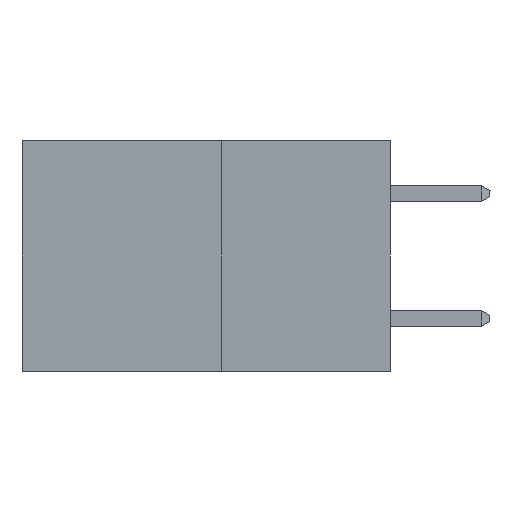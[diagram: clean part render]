
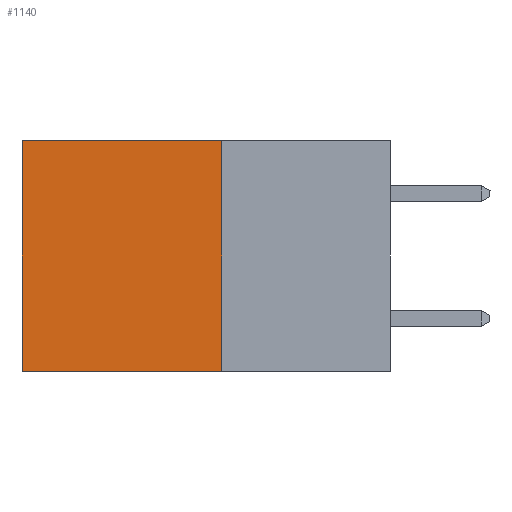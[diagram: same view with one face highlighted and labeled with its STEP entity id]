
A CAD part, left-side view. The second image highlights one B-rep face of the part: STEP entity #1140.
In plain terms, the highlighted planar face has unit normal (-1, 0, 0).
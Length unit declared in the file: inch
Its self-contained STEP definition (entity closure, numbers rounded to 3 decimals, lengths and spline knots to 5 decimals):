
#86 = CARTESIAN_POINT ( 'NONE',  ( 0.277, 0.59, -0.37 ) ) ;
#285 = CARTESIAN_POINT ( 'NONE',  ( 0.277, 0.27, 0. ) ) ;
#1140 = ADVANCED_FACE ( 'NONE', ( #10723 ), #2775, .F. ) ;
#1221 = VECTOR ( 'NONE', #5874, 39.37008 ) ;
#1782 = EDGE_CURVE ( 'NONE', #11615, #2696, #5138, .T. ) ;
#1814 = CARTESIAN_POINT ( 'NONE',  ( 0.277, 0.59, 0. ) ) ;
#1834 = ORIENTED_EDGE ( 'NONE', *, *, #4862, .T. ) ;
#2696 = VERTEX_POINT ( 'NONE', #1814 ) ;
#2775 = PLANE ( 'NONE',  #9200 ) ;
#2791 = EDGE_CURVE ( 'NONE', #6132, #6072, #4108, .T. ) ;
#2902 = CARTESIAN_POINT ( 'NONE',  ( 0.277, 0.27, -0.37 ) ) ;
#4064 = ORIENTED_EDGE ( 'NONE', *, *, #2791, .F. ) ;
#4078 = ORIENTED_EDGE ( 'NONE', *, *, #4634, .F. ) ;
#4108 = LINE ( 'NONE', #11691, #8638 ) ;
#4379 = VECTOR ( 'NONE', #5209, 39.37008 ) ;
#4634 = EDGE_CURVE ( 'NONE', #11615, #6132, #10956, .T. ) ;
#4862 = EDGE_CURVE ( 'NONE', #2696, #6072, #6765, .T. ) ;
#5138 = LINE ( 'NONE', #11269, #7789 ) ;
#5209 = DIRECTION ( 'NONE',  ( 0., 0., -1. ) ) ;
#5372 = ORIENTED_EDGE ( 'NONE', *, *, #1782, .T. ) ;
#5796 = DIRECTION ( 'NONE',  ( 0., 0., -1. ) ) ;
#5811 = DIRECTION ( 'NONE',  ( 1., 0., 0. ) ) ;
#5874 = DIRECTION ( 'NONE',  ( 0., 0., -1. ) ) ;
#6072 = VERTEX_POINT ( 'NONE', #10828 ) ;
#6132 = VERTEX_POINT ( 'NONE', #9232 ) ;
#6765 = LINE ( 'NONE', #86, #4379 ) ;
#7789 = VECTOR ( 'NONE', #10602, 39.37008 ) ;
#8638 = VECTOR ( 'NONE', #11656, 39.37008 ) ;
#9200 = AXIS2_PLACEMENT_3D ( 'NONE', #2902, #5811, #5796 ) ;
#9232 = CARTESIAN_POINT ( 'NONE',  ( 0.277, 0.27, -0.37 ) ) ;
#10241 = CARTESIAN_POINT ( 'NONE',  ( 0.277, 0.27, -0.37 ) ) ;
#10602 = DIRECTION ( 'NONE',  ( 0., 1., 0. ) ) ;
#10723 = FACE_OUTER_BOUND ( 'NONE', #10916, .T. ) ;
#10828 = CARTESIAN_POINT ( 'NONE',  ( 0.277, 0.59, -0.37 ) ) ;
#10916 = EDGE_LOOP ( 'NONE', ( #1834, #4064, #4078, #5372 ) ) ;
#10956 = LINE ( 'NONE', #10241, #1221 ) ;
#11269 = CARTESIAN_POINT ( 'NONE',  ( 0.277, 0.27, 0. ) ) ;
#11615 = VERTEX_POINT ( 'NONE', #285 ) ;
#11656 = DIRECTION ( 'NONE',  ( 0., 1., 0. ) ) ;
#11691 = CARTESIAN_POINT ( 'NONE',  ( 0.277, 0.27, -0.37 ) ) ;
